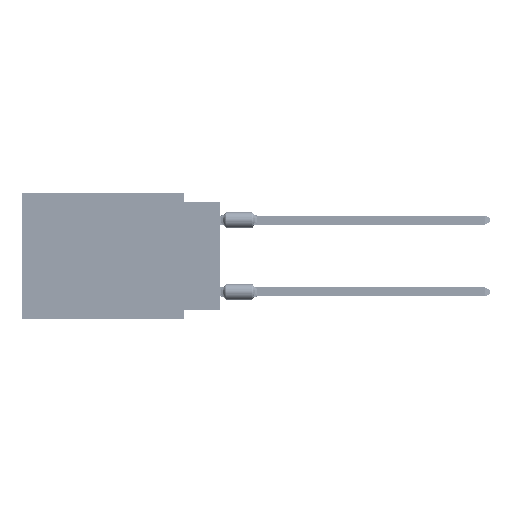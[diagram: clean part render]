
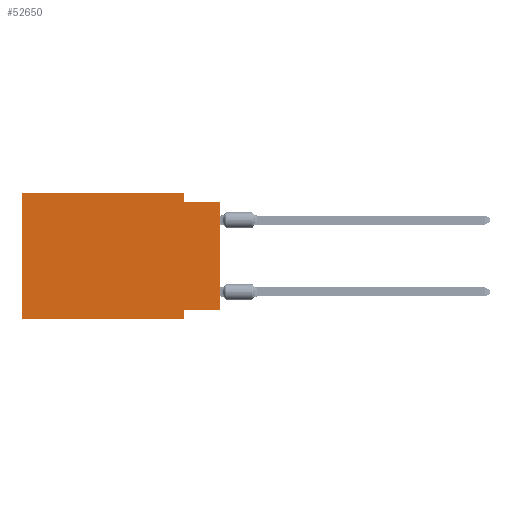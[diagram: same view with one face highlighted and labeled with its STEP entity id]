
A CAD part, left-side view. The second image highlights one B-rep face of the part: STEP entity #52650.
In plain terms, the highlighted planar face has unit normal (-1, 0, 0).
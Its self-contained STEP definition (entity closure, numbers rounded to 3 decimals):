
#2553 = CARTESIAN_POINT ( 'NONE',  ( 0., 2.54, -8.255 ) ) ;
#2987 = LINE ( 'NONE', #62084, #64082 ) ;
#4236 = AXIS2_PLACEMENT_3D ( 'NONE', #37302, #66817, #48581 ) ;
#8630 = EDGE_CURVE ( 'NONE', #74086, #67753, #2987, .T. ) ;
#8773 = VERTEX_POINT ( 'NONE', #33704 ) ;
#8804 = DIRECTION ( 'NONE',  ( 0., 0., -1. ) ) ;
#9382 = CARTESIAN_POINT ( 'NONE',  ( 0., 0., -0.635 ) ) ;
#10311 = EDGE_CURVE ( 'NONE', #67753, #54635, #75583, .T. ) ;
#11409 = VECTOR ( 'NONE', #36356, 1000. ) ;
#12091 = EDGE_LOOP ( 'NONE', ( #38401, #63301, #42054, #16517, #53074, #59546, #16446, #28693 ) ) ;
#12995 = CARTESIAN_POINT ( 'NONE',  ( 0., 13.97, 0. ) ) ;
#14717 = VECTOR ( 'NONE', #64137, 1000. ) ;
#16446 = ORIENTED_EDGE ( 'NONE', *, *, #51984, .F. ) ;
#16517 = ORIENTED_EDGE ( 'NONE', *, *, #65314, .F. ) ;
#20718 = CARTESIAN_POINT ( 'NONE',  ( 0., 2.54, 0. ) ) ;
#21939 = VECTOR ( 'NONE', #49568, 1000. ) ;
#22469 = CARTESIAN_POINT ( 'NONE',  ( 0., 0., -8.255 ) ) ;
#24817 = PLANE ( 'NONE',  #4236 ) ;
#26552 = VECTOR ( 'NONE', #43351, 1000. ) ;
#27319 = LINE ( 'NONE', #57278, #47219 ) ;
#28358 = LINE ( 'NONE', #52097, #14717 ) ;
#28478 = DIRECTION ( 'NONE',  ( 0., -1., 0. ) ) ;
#28693 = ORIENTED_EDGE ( 'NONE', *, *, #50102, .F. ) ;
#28767 = CARTESIAN_POINT ( 'NONE',  ( 0., 2.54, -8.89 ) ) ;
#29171 = VERTEX_POINT ( 'NONE', #28767 ) ;
#29854 = EDGE_CURVE ( 'NONE', #48789, #29171, #75913, .T. ) ;
#32050 = CARTESIAN_POINT ( 'NONE',  ( 0., 13.97, 0. ) ) ;
#33704 = CARTESIAN_POINT ( 'NONE',  ( 0., 13.97, 0. ) ) ;
#36356 = DIRECTION ( 'NONE',  ( 0., -1., 0. ) ) ;
#36753 = LINE ( 'NONE', #42972, #26552 ) ;
#37302 = CARTESIAN_POINT ( 'NONE',  ( 0., 13.97, 0. ) ) ;
#38401 = ORIENTED_EDGE ( 'NONE', *, *, #75538, .T. ) ;
#40557 = CARTESIAN_POINT ( 'NONE',  ( 0., 13.97, -8.89 ) ) ;
#42054 = ORIENTED_EDGE ( 'NONE', *, *, #8630, .F. ) ;
#42972 = CARTESIAN_POINT ( 'NONE',  ( 0., 0., 0. ) ) ;
#43351 = DIRECTION ( 'NONE',  ( 0., 0., 1. ) ) ;
#47219 = VECTOR ( 'NONE', #68924, 1000. ) ;
#48581 = DIRECTION ( 'NONE',  ( 0., 0., -1. ) ) ;
#48789 = VERTEX_POINT ( 'NONE', #64127 ) ;
#49568 = DIRECTION ( 'NONE',  ( 0., 0., 1. ) ) ;
#50102 = EDGE_CURVE ( 'NONE', #54186, #63754, #28358, .T. ) ;
#50340 = LINE ( 'NONE', #32050, #21939 ) ;
#51984 = EDGE_CURVE ( 'NONE', #63754, #29171, #27319, .T. ) ;
#52097 = CARTESIAN_POINT ( 'NONE',  ( 0., 0., -8.255 ) ) ;
#52650 = ADVANCED_FACE ( 'NONE', ( #54781 ), #24817, .F. ) ;
#53074 = ORIENTED_EDGE ( 'NONE', *, *, #69922, .F. ) ;
#54035 = CARTESIAN_POINT ( 'NONE',  ( 0., 2.54, -0.635 ) ) ;
#54186 = VERTEX_POINT ( 'NONE', #22469 ) ;
#54635 = VERTEX_POINT ( 'NONE', #9382 ) ;
#54781 = FACE_OUTER_BOUND ( 'NONE', #12091, .T. ) ;
#57278 = CARTESIAN_POINT ( 'NONE',  ( 0., 2.54, -8.89 ) ) ;
#59546 = ORIENTED_EDGE ( 'NONE', *, *, #29854, .T. ) ;
#62084 = CARTESIAN_POINT ( 'NONE',  ( 0., 2.54, 0. ) ) ;
#62775 = DIRECTION ( 'NONE',  ( 0., -1., 0. ) ) ;
#63158 = CARTESIAN_POINT ( 'NONE',  ( 0., 0., -0.635 ) ) ;
#63301 = ORIENTED_EDGE ( 'NONE', *, *, #10311, .F. ) ;
#63754 = VERTEX_POINT ( 'NONE', #2553 ) ;
#64082 = VECTOR ( 'NONE', #8804, 1000. ) ;
#64127 = CARTESIAN_POINT ( 'NONE',  ( 0., 13.97, -8.89 ) ) ;
#64137 = DIRECTION ( 'NONE',  ( 0., 1., 0. ) ) ;
#65314 = EDGE_CURVE ( 'NONE', #8773, #74086, #71702, .T. ) ;
#66266 = VECTOR ( 'NONE', #28478, 1000. ) ;
#66711 = VECTOR ( 'NONE', #62775, 1000. ) ;
#66817 = DIRECTION ( 'NONE',  ( 1., 0., 0. ) ) ;
#67753 = VERTEX_POINT ( 'NONE', #54035 ) ;
#68924 = DIRECTION ( 'NONE',  ( 0., 0., -1. ) ) ;
#69922 = EDGE_CURVE ( 'NONE', #48789, #8773, #50340, .T. ) ;
#71702 = LINE ( 'NONE', #12995, #11409 ) ;
#74086 = VERTEX_POINT ( 'NONE', #20718 ) ;
#75538 = EDGE_CURVE ( 'NONE', #54186, #54635, #36753, .T. ) ;
#75583 = LINE ( 'NONE', #63158, #66711 ) ;
#75913 = LINE ( 'NONE', #40557, #66266 ) ;
